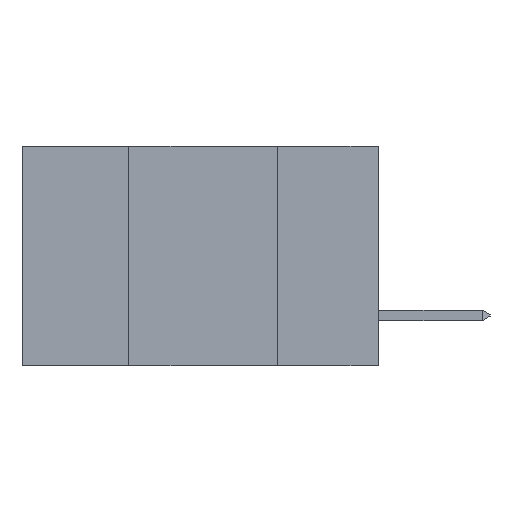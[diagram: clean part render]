
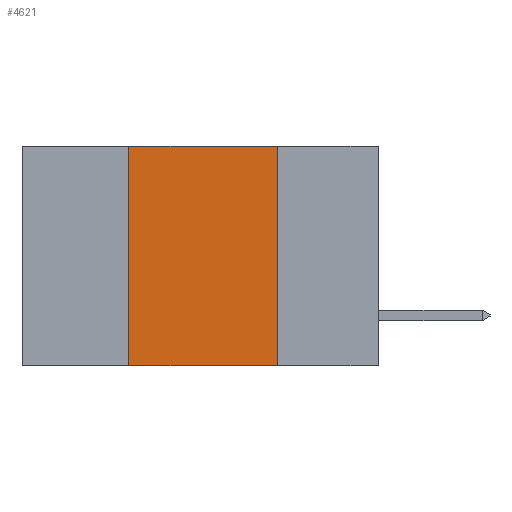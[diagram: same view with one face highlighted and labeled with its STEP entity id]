
A CAD part, left-side view. The second image highlights one B-rep face of the part: STEP entity #4621.
In plain terms, the highlighted planar face has unit normal (-1, 0, 0).
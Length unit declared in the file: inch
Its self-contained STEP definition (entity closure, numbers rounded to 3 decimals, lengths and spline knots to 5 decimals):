
#336 = DIRECTION ( 'NONE',  ( 1., 0., 0. ) ) ;
#361 = PLANE ( 'NONE',  #658 ) ;
#658 = AXIS2_PLACEMENT_3D ( 'NONE', #1025, #336, #6197 ) ;
#1025 = CARTESIAN_POINT ( 'NONE',  ( 0., 0.6, 0. ) ) ;
#1128 = CARTESIAN_POINT ( 'NONE',  ( 0., 0.42, 0. ) ) ;
#1228 = CARTESIAN_POINT ( 'NONE',  ( 0., 0.17, 0. ) ) ;
#1579 = CARTESIAN_POINT ( 'NONE',  ( 0., 0.42, -0.37 ) ) ;
#1637 = ORIENTED_EDGE ( 'NONE', *, *, #17054, .F. ) ;
#2248 = ORIENTED_EDGE ( 'NONE', *, *, #20337, .F. ) ;
#2504 = VERTEX_POINT ( 'NONE', #1579 ) ;
#3659 = CARTESIAN_POINT ( 'NONE',  ( 0., 0.6, 0. ) ) ;
#4621 = ADVANCED_FACE ( 'NONE', ( #12912 ), #361, .F. ) ;
#4767 = DIRECTION ( 'NONE',  ( 0., -1., 0. ) ) ;
#4993 = CARTESIAN_POINT ( 'NONE',  ( 0., 0.17, 0. ) ) ;
#6197 = DIRECTION ( 'NONE',  ( 0., 0., -1. ) ) ;
#7260 = VERTEX_POINT ( 'NONE', #1228 ) ;
#7878 = VERTEX_POINT ( 'NONE', #1128 ) ;
#8789 = EDGE_LOOP ( 'NONE', ( #2248, #20951, #1637, #20378 ) ) ;
#9243 = CARTESIAN_POINT ( 'NONE',  ( 0., 0.42, 0. ) ) ;
#9663 = LINE ( 'NONE', #17404, #10238 ) ;
#10238 = VECTOR ( 'NONE', #4767, 39.37008 ) ;
#11074 = VECTOR ( 'NONE', #19428, 39.37008 ) ;
#12299 = EDGE_CURVE ( 'NONE', #2504, #19838, #9663, .T. ) ;
#12912 = FACE_OUTER_BOUND ( 'NONE', #8789, .T. ) ;
#13369 = EDGE_CURVE ( 'NONE', #7878, #7260, #20149, .T. ) ;
#13704 = VECTOR ( 'NONE', #16439, 39.37008 ) ;
#14541 = DIRECTION ( 'NONE',  ( 0., -1., 0. ) ) ;
#15104 = CARTESIAN_POINT ( 'NONE',  ( 0., 0.17, -0.37 ) ) ;
#15956 = VECTOR ( 'NONE', #14541, 39.37008 ) ;
#16439 = DIRECTION ( 'NONE',  ( 0., 0., 1. ) ) ;
#17054 = EDGE_CURVE ( 'NONE', #2504, #7878, #19012, .T. ) ;
#17404 = CARTESIAN_POINT ( 'NONE',  ( 0., 0.6, -0.37 ) ) ;
#19012 = LINE ( 'NONE', #9243, #13704 ) ;
#19428 = DIRECTION ( 'NONE',  ( 0., 0., -1. ) ) ;
#19838 = VERTEX_POINT ( 'NONE', #15104 ) ;
#20149 = LINE ( 'NONE', #3659, #15956 ) ;
#20337 = EDGE_CURVE ( 'NONE', #7260, #19838, #20577, .T. ) ;
#20378 = ORIENTED_EDGE ( 'NONE', *, *, #12299, .T. ) ;
#20577 = LINE ( 'NONE', #4993, #11074 ) ;
#20951 = ORIENTED_EDGE ( 'NONE', *, *, #13369, .F. ) ;
